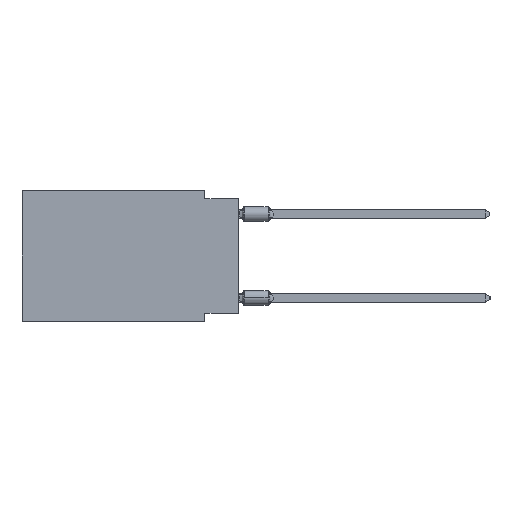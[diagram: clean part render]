
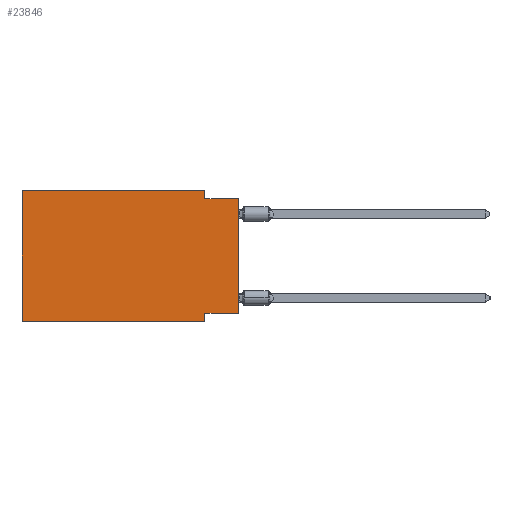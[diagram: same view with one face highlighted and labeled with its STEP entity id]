
A CAD part, left-side view. The second image highlights one B-rep face of the part: STEP entity #23846.
In plain terms, the highlighted planar face has unit normal (-1, 0, 0).
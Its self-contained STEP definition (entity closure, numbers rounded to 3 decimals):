
#721 = ORIENTED_EDGE ( 'NONE', *, *, #55149, .F. ) ;
#723 = DIRECTION ( 'NONE',  ( 0., 1., 0. ) ) ;
#1587 = LINE ( 'NONE', #53848, #37338 ) ;
#1861 = DIRECTION ( 'NONE',  ( 1., 0., 0. ) ) ;
#3718 = CARTESIAN_POINT ( 'NONE',  ( 0., 16.383, 0. ) ) ;
#5835 = VERTEX_POINT ( 'NONE', #22883 ) ;
#6183 = LINE ( 'NONE', #17250, #47262 ) ;
#7617 = VERTEX_POINT ( 'NONE', #8379 ) ;
#8379 = CARTESIAN_POINT ( 'NONE',  ( 0., 2.54, -0.635 ) ) ;
#9375 = AXIS2_PLACEMENT_3D ( 'NONE', #52793, #1861, #22337 ) ;
#9475 = VERTEX_POINT ( 'NONE', #43145 ) ;
#13670 = LINE ( 'NONE', #45471, #40341 ) ;
#15111 = VERTEX_POINT ( 'NONE', #49988 ) ;
#17170 = LINE ( 'NONE', #37580, #40003 ) ;
#17250 = CARTESIAN_POINT ( 'NONE',  ( 0., 2.54, -9.906 ) ) ;
#17363 = DIRECTION ( 'NONE',  ( 0., -1., 0. ) ) ;
#19144 = VERTEX_POINT ( 'NONE', #49013 ) ;
#20512 = ORIENTED_EDGE ( 'NONE', *, *, #40085, .F. ) ;
#21189 = CARTESIAN_POINT ( 'NONE',  ( 0., 0., -9.271 ) ) ;
#21273 = VERTEX_POINT ( 'NONE', #38940 ) ;
#21596 = DIRECTION ( 'NONE',  ( 0., 0., 1. ) ) ;
#21812 = VECTOR ( 'NONE', #35510, 1000. ) ;
#22337 = DIRECTION ( 'NONE',  ( 0., 0., -1. ) ) ;
#22883 = CARTESIAN_POINT ( 'NONE',  ( 0., 2.54, -9.271 ) ) ;
#23532 = EDGE_CURVE ( 'NONE', #21273, #50542, #13670, .T. ) ;
#23846 = ADVANCED_FACE ( 'NONE', ( #33023 ), #32361, .F. ) ;
#24207 = CARTESIAN_POINT ( 'NONE',  ( 0., 2.54, 0. ) ) ;
#25715 = CARTESIAN_POINT ( 'NONE',  ( 0., 16.383, -9.906 ) ) ;
#26548 = EDGE_CURVE ( 'NONE', #15111, #19144, #41021, .T. ) ;
#28798 = VECTOR ( 'NONE', #52052, 1000. ) ;
#31964 = CARTESIAN_POINT ( 'NONE',  ( 0., 0., 0. ) ) ;
#32361 = PLANE ( 'NONE',  #9375 ) ;
#32560 = LINE ( 'NONE', #21189, #50567 ) ;
#33023 = FACE_OUTER_BOUND ( 'NONE', #58579, .T. ) ;
#33339 = EDGE_CURVE ( 'NONE', #15111, #5835, #32560, .T. ) ;
#35510 = DIRECTION ( 'NONE',  ( 0., 0., 1. ) ) ;
#36534 = VERTEX_POINT ( 'NONE', #25715 ) ;
#37338 = VECTOR ( 'NONE', #17363, 1000. ) ;
#37580 = CARTESIAN_POINT ( 'NONE',  ( 0., 2.54, 0. ) ) ;
#37656 = DIRECTION ( 'NONE',  ( 0., 0., -1. ) ) ;
#38940 = CARTESIAN_POINT ( 'NONE',  ( 0., 16.383, 0. ) ) ;
#39791 = ORIENTED_EDGE ( 'NONE', *, *, #26548, .T. ) ;
#40003 = VECTOR ( 'NONE', #58033, 1000. ) ;
#40085 = EDGE_CURVE ( 'NONE', #7617, #19144, #1587, .T. ) ;
#40341 = VECTOR ( 'NONE', #59241, 1000. ) ;
#41021 = LINE ( 'NONE', #31964, #50104 ) ;
#43145 = CARTESIAN_POINT ( 'NONE',  ( 0., 2.54, -9.906 ) ) ;
#45471 = CARTESIAN_POINT ( 'NONE',  ( 0., 16.383, 0. ) ) ;
#47071 = ORIENTED_EDGE ( 'NONE', *, *, #64552, .T. ) ;
#47262 = VECTOR ( 'NONE', #37656, 1000. ) ;
#47489 = EDGE_CURVE ( 'NONE', #50542, #7617, #17170, .T. ) ;
#47762 = ORIENTED_EDGE ( 'NONE', *, *, #33339, .F. ) ;
#49013 = CARTESIAN_POINT ( 'NONE',  ( 0., 0., -0.635 ) ) ;
#49988 = CARTESIAN_POINT ( 'NONE',  ( 0., 0., -9.271 ) ) ;
#50104 = VECTOR ( 'NONE', #21596, 1000. ) ;
#50542 = VERTEX_POINT ( 'NONE', #24207 ) ;
#50567 = VECTOR ( 'NONE', #723, 1000. ) ;
#51071 = CARTESIAN_POINT ( 'NONE',  ( 0., 16.383, -9.906 ) ) ;
#52052 = DIRECTION ( 'NONE',  ( 0., -1., 0. ) ) ;
#52198 = EDGE_CURVE ( 'NONE', #5835, #9475, #6183, .T. ) ;
#52793 = CARTESIAN_POINT ( 'NONE',  ( 0., 16.383, 0. ) ) ;
#53848 = CARTESIAN_POINT ( 'NONE',  ( 0., 0., -0.635 ) ) ;
#55149 = EDGE_CURVE ( 'NONE', #36534, #21273, #59990, .T. ) ;
#55527 = ORIENTED_EDGE ( 'NONE', *, *, #23532, .F. ) ;
#57246 = ORIENTED_EDGE ( 'NONE', *, *, #52198, .F. ) ;
#58033 = DIRECTION ( 'NONE',  ( 0., 0., -1. ) ) ;
#58579 = EDGE_LOOP ( 'NONE', ( #39791, #20512, #58740, #55527, #721, #47071, #57246, #47762 ) ) ;
#58740 = ORIENTED_EDGE ( 'NONE', *, *, #47489, .F. ) ;
#59241 = DIRECTION ( 'NONE',  ( 0., -1., 0. ) ) ;
#59990 = LINE ( 'NONE', #3718, #21812 ) ;
#61784 = LINE ( 'NONE', #51071, #28798 ) ;
#64552 = EDGE_CURVE ( 'NONE', #36534, #9475, #61784, .T. ) ;
